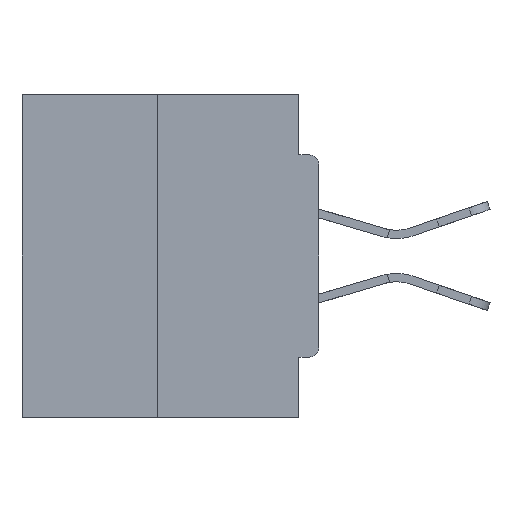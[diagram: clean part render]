
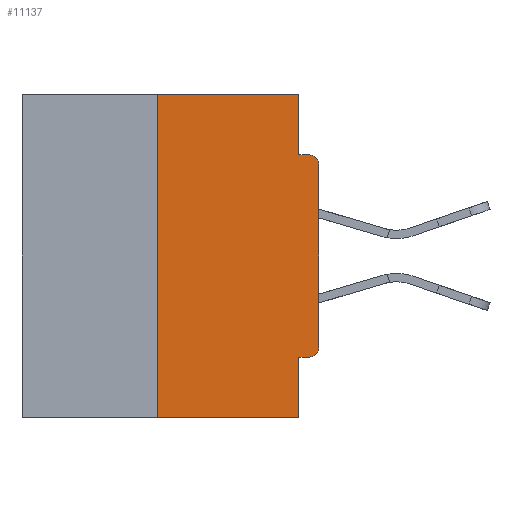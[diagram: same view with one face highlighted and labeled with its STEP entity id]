
A CAD part, left-side view. The second image highlights one B-rep face of the part: STEP entity #11137.
In plain terms, the highlighted planar face has unit normal (-1, 0, 0).
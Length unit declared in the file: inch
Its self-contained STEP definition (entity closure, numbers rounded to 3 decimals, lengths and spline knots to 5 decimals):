
#283 = DIRECTION ( 'NONE',  ( 1., 0., 0. ) ) ;
#520 = EDGE_CURVE ( 'NONE', #6478, #32714, #9579, .T. ) ;
#781 = CARTESIAN_POINT ( 'NONE',  ( 0., 0.015, -0.1085 ) ) ;
#1036 = LINE ( 'NONE', #23624, #14567 ) ;
#1284 = VERTEX_POINT ( 'NONE', #2193 ) ;
#1565 = AXIS2_PLACEMENT_3D ( 'NONE', #781, #16730, #11408 ) ;
#1946 = DIRECTION ( 'NONE',  ( 0., 0., 1. ) ) ;
#2193 = CARTESIAN_POINT ( 'NONE',  ( 0., 0.25, -0.5 ) ) ;
#2290 = EDGE_CURVE ( 'NONE', #1284, #3255, #9595, .T. ) ;
#2910 = CARTESIAN_POINT ( 'NONE',  ( 0., 0.015, -0.3915 ) ) ;
#3143 = VECTOR ( 'NONE', #21414, 39.37008 ) ;
#3255 = VERTEX_POINT ( 'NONE', #4786 ) ;
#3805 = LINE ( 'NONE', #34429, #26231 ) ;
#4371 = CARTESIAN_POINT ( 'NONE',  ( 0., 0.015, -0.4065 ) ) ;
#4451 = EDGE_CURVE ( 'NONE', #6478, #26444, #5249, .T. ) ;
#4538 = CIRCLE ( 'NONE', #1565, 0.015 ) ;
#4786 = CARTESIAN_POINT ( 'NONE',  ( 0., 0.031, -0.5 ) ) ;
#4860 = CARTESIAN_POINT ( 'NONE',  ( 0., 0.031, -0.5 ) ) ;
#5067 = DIRECTION ( 'NONE',  ( 0., -1., 0. ) ) ;
#5249 = LINE ( 'NONE', #8452, #9866 ) ;
#5252 = CARTESIAN_POINT ( 'NONE',  ( 0., 0.031, -0.0935 ) ) ;
#5381 = CARTESIAN_POINT ( 'NONE',  ( 0., 0., 0. ) ) ;
#6478 = VERTEX_POINT ( 'NONE', #4371 ) ;
#6738 = ORIENTED_EDGE ( 'NONE', *, *, #10431, .T. ) ;
#7296 = VECTOR ( 'NONE', #8403, 39.37008 ) ;
#7775 = EDGE_CURVE ( 'NONE', #32289, #29536, #4538, .T. ) ;
#8403 = DIRECTION ( 'NONE',  ( 0., 0., 1. ) ) ;
#8411 = ORIENTED_EDGE ( 'NONE', *, *, #520, .T. ) ;
#8452 = CARTESIAN_POINT ( 'NONE',  ( 0., 0., -0.4065 ) ) ;
#8485 = VERTEX_POINT ( 'NONE', #31799 ) ;
#9183 = CARTESIAN_POINT ( 'NONE',  ( 0., 0.46, -0.5 ) ) ;
#9579 = CIRCLE ( 'NONE', #13888, 0.015 ) ;
#9595 = LINE ( 'NONE', #9183, #18519 ) ;
#9866 = VECTOR ( 'NONE', #30357, 39.37008 ) ;
#10046 = EDGE_CURVE ( 'NONE', #23938, #8485, #26354, .T. ) ;
#10431 = EDGE_CURVE ( 'NONE', #32714, #32289, #17444, .T. ) ;
#11137 = ADVANCED_FACE ( 'NONE', ( #23269 ), #16571, .F. ) ;
#11408 = DIRECTION ( 'NONE',  ( 0., 0., -1. ) ) ;
#11623 = ORIENTED_EDGE ( 'NONE', *, *, #4451, .F. ) ;
#13032 = DIRECTION ( 'NONE',  ( 0., -1., 0. ) ) ;
#13888 = AXIS2_PLACEMENT_3D ( 'NONE', #2910, #18494, #21811 ) ;
#14567 = VECTOR ( 'NONE', #5067, 39.37008 ) ;
#15639 = ORIENTED_EDGE ( 'NONE', *, *, #30758, .F. ) ;
#16333 = AXIS2_PLACEMENT_3D ( 'NONE', #27109, #283, #32872 ) ;
#16571 = PLANE ( 'NONE',  #16333 ) ;
#16601 = CARTESIAN_POINT ( 'NONE',  ( 0., 0., -0.1085 ) ) ;
#16730 = DIRECTION ( 'NONE',  ( -1., 0., 0. ) ) ;
#17365 = CARTESIAN_POINT ( 'NONE',  ( 0., 0.25, 0. ) ) ;
#17437 = ORIENTED_EDGE ( 'NONE', *, *, #2290, .T. ) ;
#17444 = LINE ( 'NONE', #5381, #7296 ) ;
#17756 = CARTESIAN_POINT ( 'NONE',  ( 0., 0.25, 0. ) ) ;
#18494 = DIRECTION ( 'NONE',  ( -1., 0., 0. ) ) ;
#18519 = VECTOR ( 'NONE', #28014, 39.37008 ) ;
#18590 = LINE ( 'NONE', #17756, #34213 ) ;
#20296 = CARTESIAN_POINT ( 'NONE',  ( 0., 0., -0.3915 ) ) ;
#20420 = CARTESIAN_POINT ( 'NONE',  ( 0., 0.015, -0.0935 ) ) ;
#21414 = DIRECTION ( 'NONE',  ( 0., 0., -1. ) ) ;
#21645 = VERTEX_POINT ( 'NONE', #5252 ) ;
#21811 = DIRECTION ( 'NONE',  ( 0., 0., -1. ) ) ;
#22842 = EDGE_CURVE ( 'NONE', #26444, #3255, #33991, .T. ) ;
#23269 = FACE_OUTER_BOUND ( 'NONE', #32616, .T. ) ;
#23624 = CARTESIAN_POINT ( 'NONE',  ( 0., 0., -0.0935 ) ) ;
#23938 = VERTEX_POINT ( 'NONE', #17365 ) ;
#24670 = ORIENTED_EDGE ( 'NONE', *, *, #27491, .F. ) ;
#25904 = ORIENTED_EDGE ( 'NONE', *, *, #7775, .T. ) ;
#26231 = VECTOR ( 'NONE', #34300, 39.37008 ) ;
#26285 = ORIENTED_EDGE ( 'NONE', *, *, #22842, .F. ) ;
#26354 = LINE ( 'NONE', #34518, #33932 ) ;
#26444 = VERTEX_POINT ( 'NONE', #28119 ) ;
#27109 = CARTESIAN_POINT ( 'NONE',  ( 0., 0.46, 0. ) ) ;
#27491 = EDGE_CURVE ( 'NONE', #21645, #29536, #1036, .T. ) ;
#28014 = DIRECTION ( 'NONE',  ( 0., -1., 0. ) ) ;
#28119 = CARTESIAN_POINT ( 'NONE',  ( 0., 0.031, -0.4065 ) ) ;
#28246 = ORIENTED_EDGE ( 'NONE', *, *, #10046, .F. ) ;
#29536 = VERTEX_POINT ( 'NONE', #20420 ) ;
#30261 = EDGE_CURVE ( 'NONE', #8485, #21645, #3805, .T. ) ;
#30357 = DIRECTION ( 'NONE',  ( 0., 1., 0. ) ) ;
#30758 = EDGE_CURVE ( 'NONE', #1284, #23938, #18590, .T. ) ;
#31799 = CARTESIAN_POINT ( 'NONE',  ( 0., 0.031, 0. ) ) ;
#31903 = ORIENTED_EDGE ( 'NONE', *, *, #30261, .F. ) ;
#32289 = VERTEX_POINT ( 'NONE', #16601 ) ;
#32616 = EDGE_LOOP ( 'NONE', ( #28246, #15639, #17437, #26285, #11623, #8411, #6738, #25904, #24670, #31903 ) ) ;
#32714 = VERTEX_POINT ( 'NONE', #20296 ) ;
#32872 = DIRECTION ( 'NONE',  ( 0., 0., -1. ) ) ;
#33932 = VECTOR ( 'NONE', #13032, 39.37008 ) ;
#33991 = LINE ( 'NONE', #4860, #3143 ) ;
#34213 = VECTOR ( 'NONE', #1946, 39.37008 ) ;
#34300 = DIRECTION ( 'NONE',  ( 0., 0., -1. ) ) ;
#34429 = CARTESIAN_POINT ( 'NONE',  ( 0., 0.031, 0. ) ) ;
#34518 = CARTESIAN_POINT ( 'NONE',  ( 0., 0.46, 0. ) ) ;
